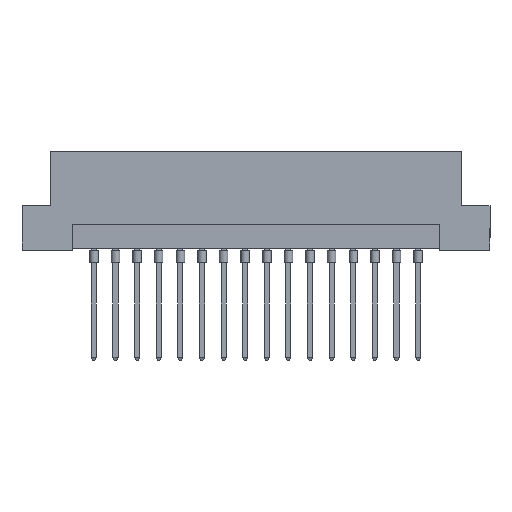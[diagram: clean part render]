
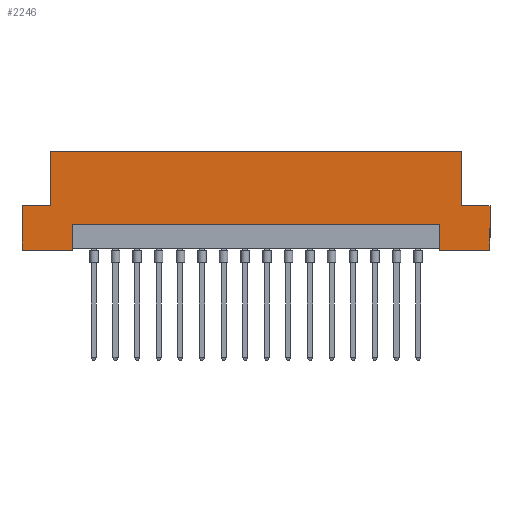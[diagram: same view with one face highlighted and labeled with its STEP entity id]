
A CAD part, front view. The second image highlights one B-rep face of the part: STEP entity #2246.
In plain terms, the highlighted planar face has unit normal (0, -1, 0).
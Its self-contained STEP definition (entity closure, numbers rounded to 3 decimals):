
#12 = EDGE_CURVE ( 'NONE', #3942, #7119, #4603, .T. ) ;
#35 = VERTEX_POINT ( 'NONE', #6344 ) ;
#248 = ORIENTED_EDGE ( 'NONE', *, *, #4326, .T. ) ;
#381 = VECTOR ( 'NONE', #1557, 1000. ) ;
#478 = CARTESIAN_POINT ( 'NONE',  ( -27.5, -4.3, 0. ) ) ;
#499 = LINE ( 'NONE', #4101, #5425 ) ;
#517 = DIRECTION ( 'NONE',  ( 1., 0., 0. ) ) ;
#523 = VERTEX_POINT ( 'NONE', #5674 ) ;
#607 = CARTESIAN_POINT ( 'NONE',  ( 27.5, -4.3, 11.6 ) ) ;
#646 = EDGE_CURVE ( 'NONE', #4167, #523, #1635, .T. ) ;
#798 = AXIS2_PLACEMENT_3D ( 'NONE', #6411, #3501, #4081 ) ;
#926 = CARTESIAN_POINT ( 'NONE',  ( 27.5, -4.3, 5.2 ) ) ;
#975 = EDGE_CURVE ( 'NONE', #7074, #7410, #1548, .T. ) ;
#1018 = CARTESIAN_POINT ( 'NONE',  ( -24.2, -4.3, 11.6 ) ) ;
#1044 = CARTESIAN_POINT ( 'NONE',  ( -21.6, -4.3, 3. ) ) ;
#1238 = VERTEX_POINT ( 'NONE', #7137 ) ;
#1548 = LINE ( 'NONE', #3260, #2801 ) ;
#1552 = CARTESIAN_POINT ( 'NONE',  ( 24.2, -4.3, 5.2 ) ) ;
#1557 = DIRECTION ( 'NONE',  ( 1., 0., 0. ) ) ;
#1558 = VECTOR ( 'NONE', #5777, 1000. ) ;
#1610 = DIRECTION ( 'NONE',  ( 1., 0., 0. ) ) ;
#1635 = LINE ( 'NONE', #1044, #4474 ) ;
#1652 = CARTESIAN_POINT ( 'NONE',  ( 21.6, -4.3, 0.2 ) ) ;
#1655 = EDGE_CURVE ( 'NONE', #3942, #523, #2925, .T. ) ;
#1737 = CARTESIAN_POINT ( 'NONE',  ( 24.2, -4.3, 11.6 ) ) ;
#1773 = EDGE_CURVE ( 'NONE', #1238, #5231, #6703, .T. ) ;
#1825 = ORIENTED_EDGE ( 'NONE', *, *, #12, .T. ) ;
#2062 = CARTESIAN_POINT ( 'NONE',  ( -27.5, -4.3, 5.2 ) ) ;
#2246 = ADVANCED_FACE ( 'NONE', ( #2841 ), #4006, .F. ) ;
#2263 = CARTESIAN_POINT ( 'NONE',  ( 27.5, -4.3, 5.2 ) ) ;
#2563 = EDGE_CURVE ( 'NONE', #3973, #4099, #6789, .T. ) ;
#2697 = ORIENTED_EDGE ( 'NONE', *, *, #2563, .F. ) ;
#2700 = DIRECTION ( 'NONE',  ( 0., 0., -1. ) ) ;
#2753 = DIRECTION ( 'NONE',  ( 1., 0., 0. ) ) ;
#2758 = EDGE_CURVE ( 'NONE', #3973, #4733, #6908, .T. ) ;
#2786 = LINE ( 'NONE', #6403, #381 ) ;
#2801 = VECTOR ( 'NONE', #2700, 1000. ) ;
#2841 = FACE_OUTER_BOUND ( 'NONE', #3324, .T. ) ;
#2845 = ORIENTED_EDGE ( 'NONE', *, *, #1773, .F. ) ;
#2875 = ORIENTED_EDGE ( 'NONE', *, *, #975, .T. ) ;
#2925 = LINE ( 'NONE', #1652, #3192 ) ;
#2932 = VECTOR ( 'NONE', #6009, 1000. ) ;
#2983 = LINE ( 'NONE', #7263, #2932 ) ;
#3093 = DIRECTION ( 'NONE',  ( 0., 0., -1. ) ) ;
#3192 = VECTOR ( 'NONE', #7639, 1000. ) ;
#3229 = DIRECTION ( 'NONE',  ( 1., 0., 0. ) ) ;
#3230 = CARTESIAN_POINT ( 'NONE',  ( 24.2, -4.3, 5.2 ) ) ;
#3260 = CARTESIAN_POINT ( 'NONE',  ( -27.5, -4.3, 11.6 ) ) ;
#3324 = EDGE_LOOP ( 'NONE', ( #5252, #6559, #1825, #3994, #2697, #6254, #4913, #2845, #6975, #2875, #248, #4751 ) ) ;
#3481 = EDGE_CURVE ( 'NONE', #5231, #4733, #7545, .T. ) ;
#3501 = DIRECTION ( 'NONE',  ( 0., 1., 0. ) ) ;
#3675 = DIRECTION ( 'NONE',  ( 0., 0., 1. ) ) ;
#3942 = VERTEX_POINT ( 'NONE', #6870 ) ;
#3973 = VERTEX_POINT ( 'NONE', #3230 ) ;
#3994 = ORIENTED_EDGE ( 'NONE', *, *, #4885, .F. ) ;
#4006 = PLANE ( 'NONE',  #798 ) ;
#4081 = DIRECTION ( 'NONE',  ( -1., 0., 0. ) ) ;
#4099 = VERTEX_POINT ( 'NONE', #2263 ) ;
#4101 = CARTESIAN_POINT ( 'NONE',  ( -21.6, -4.3, 0.2 ) ) ;
#4167 = VERTEX_POINT ( 'NONE', #7534 ) ;
#4302 = VECTOR ( 'NONE', #3675, 1000. ) ;
#4326 = EDGE_CURVE ( 'NONE', #7410, #35, #2983, .T. ) ;
#4474 = VECTOR ( 'NONE', #517, 1000. ) ;
#4482 = CARTESIAN_POINT ( 'NONE',  ( 27.5, -4.3, 0. ) ) ;
#4603 = LINE ( 'NONE', #4482, #7321 ) ;
#4604 = EDGE_CURVE ( 'NONE', #4167, #35, #499, .T. ) ;
#4727 = DIRECTION ( 'NONE',  ( 0., 0., -1. ) ) ;
#4733 = VERTEX_POINT ( 'NONE', #1737 ) ;
#4751 = ORIENTED_EDGE ( 'NONE', *, *, #4604, .F. ) ;
#4885 = EDGE_CURVE ( 'NONE', #4099, #7119, #5968, .T. ) ;
#4913 = ORIENTED_EDGE ( 'NONE', *, *, #3481, .F. ) ;
#5231 = VERTEX_POINT ( 'NONE', #1018 ) ;
#5252 = ORIENTED_EDGE ( 'NONE', *, *, #646, .T. ) ;
#5425 = VECTOR ( 'NONE', #4727, 1000. ) ;
#5674 = CARTESIAN_POINT ( 'NONE',  ( 21.6, -4.3, 3. ) ) ;
#5777 = DIRECTION ( 'NONE',  ( 0., 0., 1. ) ) ;
#5968 = LINE ( 'NONE', #607, #6415 ) ;
#6009 = DIRECTION ( 'NONE',  ( 1., 0., 0. ) ) ;
#6254 = ORIENTED_EDGE ( 'NONE', *, *, #2758, .T. ) ;
#6344 = CARTESIAN_POINT ( 'NONE',  ( -21.6, -4.3, 0. ) ) ;
#6403 = CARTESIAN_POINT ( 'NONE',  ( -27.5, -4.3, 5.2 ) ) ;
#6411 = CARTESIAN_POINT ( 'NONE',  ( 27.5, -4.3, 11.6 ) ) ;
#6415 = VECTOR ( 'NONE', #3093, 1000. ) ;
#6543 = VECTOR ( 'NONE', #3229, 1000. ) ;
#6559 = ORIENTED_EDGE ( 'NONE', *, *, #1655, .F. ) ;
#6606 = CARTESIAN_POINT ( 'NONE',  ( 27.5, -4.3, 0. ) ) ;
#6703 = LINE ( 'NONE', #7217, #4302 ) ;
#6789 = LINE ( 'NONE', #926, #6543 ) ;
#6799 = VECTOR ( 'NONE', #2753, 1000. ) ;
#6870 = CARTESIAN_POINT ( 'NONE',  ( 21.6, -4.3, 0. ) ) ;
#6908 = LINE ( 'NONE', #1552, #1558 ) ;
#6975 = ORIENTED_EDGE ( 'NONE', *, *, #7511, .F. ) ;
#7074 = VERTEX_POINT ( 'NONE', #2062 ) ;
#7119 = VERTEX_POINT ( 'NONE', #6606 ) ;
#7137 = CARTESIAN_POINT ( 'NONE',  ( -24.2, -4.3, 5.2 ) ) ;
#7217 = CARTESIAN_POINT ( 'NONE',  ( -24.2, -4.3, 5.2 ) ) ;
#7263 = CARTESIAN_POINT ( 'NONE',  ( 27.5, -4.3, 0. ) ) ;
#7321 = VECTOR ( 'NONE', #1610, 1000. ) ;
#7410 = VERTEX_POINT ( 'NONE', #478 ) ;
#7467 = CARTESIAN_POINT ( 'NONE',  ( 27.5, -4.3, 11.6 ) ) ;
#7511 = EDGE_CURVE ( 'NONE', #7074, #1238, #2786, .T. ) ;
#7534 = CARTESIAN_POINT ( 'NONE',  ( -21.6, -4.3, 3. ) ) ;
#7545 = LINE ( 'NONE', #7467, #6799 ) ;
#7639 = DIRECTION ( 'NONE',  ( 0., 0., 1. ) ) ;
